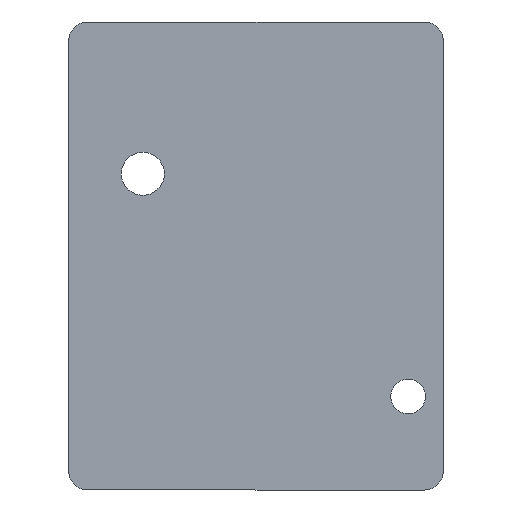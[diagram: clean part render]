
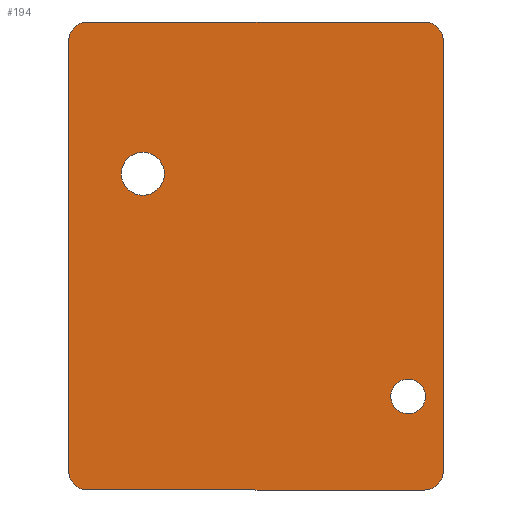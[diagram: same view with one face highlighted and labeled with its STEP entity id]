
A CAD part, front view. The second image highlights one B-rep face of the part: STEP entity #194.
In plain terms, the highlighted planar face has unit normal (0, -1, 0).
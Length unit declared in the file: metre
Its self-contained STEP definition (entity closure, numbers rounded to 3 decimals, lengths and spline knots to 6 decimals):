
#194 = ADVANCED_FACE( '', ( #398, #399, #400 ), #401, .T. );
#398 = FACE_BOUND( '', #602, .T. );
#399 = FACE_BOUND( '', #603, .T. );
#400 = FACE_OUTER_BOUND( '', #604, .T. );
#401 = PLANE( '', #605 );
#602 = EDGE_LOOP( '', ( #1113 ) );
#603 = EDGE_LOOP( '', ( #1114 ) );
#604 = EDGE_LOOP( '', ( #1115, #1116, #1117, #1118, #1119, #1120, #1121, #1122 ) );
#605 = AXIS2_PLACEMENT_3D( '', #1123, #1124, #1125 );
#1113 = ORIENTED_EDGE( '', *, *, #1347, .T. );
#1114 = ORIENTED_EDGE( '', *, *, #1360, .F. );
#1115 = ORIENTED_EDGE( '', *, *, #1262, .F. );
#1116 = ORIENTED_EDGE( '', *, *, #1314, .T. );
#1117 = ORIENTED_EDGE( '', *, *, #1212, .F. );
#1118 = ORIENTED_EDGE( '', *, *, #1241, .T. );
#1119 = ORIENTED_EDGE( '', *, *, #1400, .F. );
#1120 = ORIENTED_EDGE( '', *, *, #1217, .T. );
#1121 = ORIENTED_EDGE( '', *, *, #1329, .F. );
#1122 = ORIENTED_EDGE( '', *, *, #1302, .T. );
#1123 = CARTESIAN_POINT( '', ( 0., 0., 0. ) );
#1124 = DIRECTION( '', ( 0., -1., 0. ) );
#1125 = DIRECTION( '', ( 0., 0., -1. ) );
#1212 = EDGE_CURVE( '', #1448, #1443, #1450, .T. );
#1217 = EDGE_CURVE( '', #1453, #1457, #1459, .T. );
#1241 = EDGE_CURVE( '', #1448, #1498, #1500, .T. );
#1262 = EDGE_CURVE( '', #1535, #1537, #1538, .T. );
#1302 = EDGE_CURVE( '', #1595, #1537, #1598, .T. );
#1314 = EDGE_CURVE( '', #1535, #1443, #1614, .T. );
#1329 = EDGE_CURVE( '', #1595, #1457, #1632, .T. );
#1347 = EDGE_CURVE( '', #1655, #1655, #1656, .T. );
#1360 = EDGE_CURVE( '', #1672, #1672, #1673, .T. );
#1400 = EDGE_CURVE( '', #1453, #1498, #1721, .T. );
#1443 = VERTEX_POINT( '', #1777 );
#1448 = VERTEX_POINT( '', #1784 );
#1450 = LINE( '', #1787, #1788 );
#1453 = VERTEX_POINT( '', #1791 );
#1457 = VERTEX_POINT( '', #1796 );
#1459 = CIRCLE( '', #1799, 0.00254 );
#1498 = VERTEX_POINT( '', #1855 );
#1500 = CIRCLE( '', #1858, 0.00254 );
#1535 = VERTEX_POINT( '', #1905 );
#1537 = VERTEX_POINT( '', #1908 );
#1538 = LINE( '', #1909, #1910 );
#1595 = VERTEX_POINT( '', #1997 );
#1598 = CIRCLE( '', #2001, 0.00254 );
#1614 = CIRCLE( '', #2022, 0.00254 );
#1632 = LINE( '', #2044, #2045 );
#1655 = VERTEX_POINT( '', #2075 );
#1656 = CIRCLE( '', #2076, 0.002921 );
#1672 = VERTEX_POINT( '', #2093 );
#1673 = CIRCLE( '', #2094, 0.00235 );
#1721 = LINE( '', #2159, #2160 );
#1777 = CARTESIAN_POINT( '', ( -0.04826, 0., 0. ) );
#1784 = CARTESIAN_POINT( '', ( -0.00254, 0., 0. ) );
#1787 = CARTESIAN_POINT( '', ( 0., 0., 0. ) );
#1788 = VECTOR( '', #2191, 1. );
#1791 = CARTESIAN_POINT( '', ( 0., 0., 0.06096 ) );
#1796 = CARTESIAN_POINT( '', ( -0.00254, 0., 0.0635 ) );
#1799 = AXIS2_PLACEMENT_3D( '', #2197, #2198, #2199 );
#1855 = CARTESIAN_POINT( '', ( 0., 0., 0.00254 ) );
#1858 = AXIS2_PLACEMENT_3D( '', #2221, #2222, #2223 );
#1905 = CARTESIAN_POINT( '', ( -0.0508, 0., 0.00254 ) );
#1908 = CARTESIAN_POINT( '', ( -0.0508, 0., 0.06096 ) );
#1909 = CARTESIAN_POINT( '', ( -0.0508, 0., 0. ) );
#1910 = VECTOR( '', #2246, 1. );
#1997 = CARTESIAN_POINT( '', ( -0.04826, 0., 0.0635 ) );
#2001 = AXIS2_PLACEMENT_3D( '', #2300, #2301, #2302 );
#2022 = AXIS2_PLACEMENT_3D( '', #2314, #2315, #2316 );
#2044 = CARTESIAN_POINT( '', ( 0., 0., 0.0635 ) );
#2045 = VECTOR( '', #2336, 1. );
#2075 = CARTESIAN_POINT( '', ( -0.040759, 0., 0.045826 ) );
#2076 = AXIS2_PLACEMENT_3D( '', #2356, #2357, #2358 );
#2093 = CARTESIAN_POINT( '', ( -0.004763, 0., 0.010351 ) );
#2094 = AXIS2_PLACEMENT_3D( '', #2378, #2379, #2380 );
#2159 = CARTESIAN_POINT( '', ( 0., 0., 0. ) );
#2160 = VECTOR( '', #2419, 1. );
#2191 = DIRECTION( '', ( -1., 0., 0. ) );
#2197 = CARTESIAN_POINT( '', ( -0.00254, 0., 0.06096 ) );
#2198 = DIRECTION( '', ( 0., -1., 0. ) );
#2199 = DIRECTION( '', ( 0., 0., -1. ) );
#2221 = CARTESIAN_POINT( '', ( -0.00254, 0., 0.00254 ) );
#2222 = DIRECTION( '', ( 0., -1., 0. ) );
#2223 = DIRECTION( '', ( 0., 0., -1. ) );
#2246 = DIRECTION( '', ( 0., 0., 1. ) );
#2300 = CARTESIAN_POINT( '', ( -0.04826, 0., 0.06096 ) );
#2301 = DIRECTION( '', ( 0., -1., 0. ) );
#2302 = DIRECTION( '', ( 0., 0., -1. ) );
#2314 = CARTESIAN_POINT( '', ( -0.04826, 0., 0.00254 ) );
#2315 = DIRECTION( '', ( 0., -1., 0. ) );
#2316 = DIRECTION( '', ( 0., 0., -1. ) );
#2336 = DIRECTION( '', ( 1., 0., 0. ) );
#2356 = CARTESIAN_POINT( '', ( -0.040759, 0., 0.042905 ) );
#2357 = DIRECTION( '', ( 0., 1., 0. ) );
#2358 = DIRECTION( '', ( 0., 0., 1. ) );
#2378 = CARTESIAN_POINT( '', ( -0.004763, 0., 0.0127 ) );
#2379 = DIRECTION( '', ( 0., -1., 0. ) );
#2380 = DIRECTION( '', ( 0., 0., -1. ) );
#2419 = DIRECTION( '', ( 0., 0., -1. ) );
